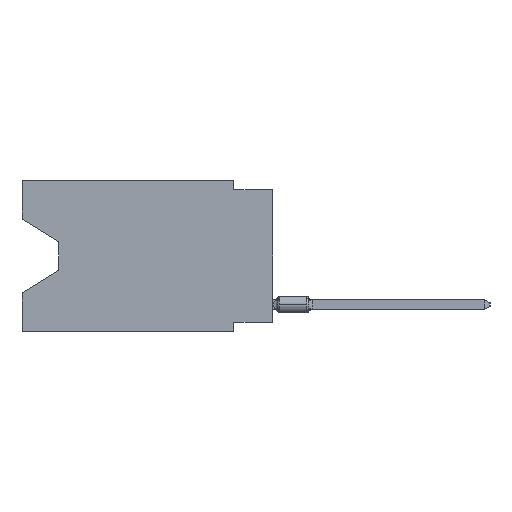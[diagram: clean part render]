
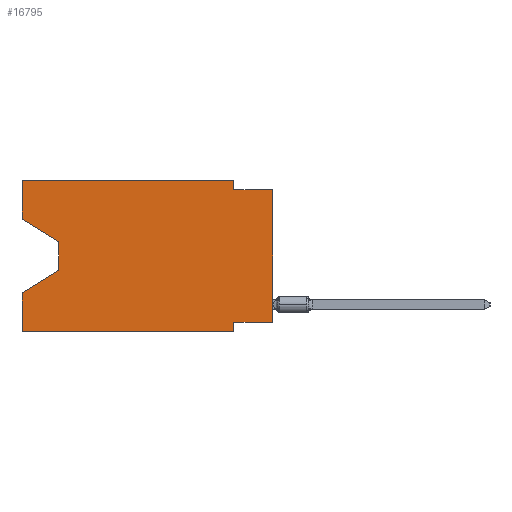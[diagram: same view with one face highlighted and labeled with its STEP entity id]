
A CAD part, left-side view. The second image highlights one B-rep face of the part: STEP entity #16795.
In plain terms, the highlighted planar face has unit normal (-1, 0, 0).
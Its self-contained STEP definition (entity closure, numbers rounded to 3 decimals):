
#233 = CARTESIAN_POINT ( 'NONE',  ( 0., 0., -0.635 ) ) ;
#667 = DIRECTION ( 'NONE',  ( 0., 0., -1. ) ) ;
#679 = EDGE_CURVE ( 'NONE', #49592, #24781, #42733, .T. ) ;
#1948 = CARTESIAN_POINT ( 'NONE',  ( 0., 16.383, -9.906 ) ) ;
#2974 = VERTEX_POINT ( 'NONE', #40757 ) ;
#4372 = CARTESIAN_POINT ( 'NONE',  ( 0., 0., -0.635 ) ) ;
#4913 = CARTESIAN_POINT ( 'NONE',  ( 0., 16.383, -9.906 ) ) ;
#5333 = CARTESIAN_POINT ( 'NONE',  ( 0., 16.383, -7.36 ) ) ;
#5532 = VECTOR ( 'NONE', #49295, 1000. ) ;
#6837 = ORIENTED_EDGE ( 'NONE', *, *, #34905, .T. ) ;
#8085 = ORIENTED_EDGE ( 'NONE', *, *, #13207, .F. ) ;
#9167 = VERTEX_POINT ( 'NONE', #4372 ) ;
#9658 = DIRECTION ( 'NONE',  ( 0., 0.855, -0.519 ) ) ;
#9728 = DIRECTION ( 'NONE',  ( 1., 0., 0. ) ) ;
#9980 = VERTEX_POINT ( 'NONE', #48731 ) ;
#10377 = CARTESIAN_POINT ( 'NONE',  ( 0., 0., -9.271 ) ) ;
#10813 = CARTESIAN_POINT ( 'NONE',  ( 0., 2.54, 0. ) ) ;
#10932 = EDGE_CURVE ( 'NONE', #11700, #13028, #24825, .T. ) ;
#11700 = VERTEX_POINT ( 'NONE', #32693 ) ;
#12869 = AXIS2_PLACEMENT_3D ( 'NONE', #33815, #9728, #41316 ) ;
#13028 = VERTEX_POINT ( 'NONE', #39754 ) ;
#13207 = EDGE_CURVE ( 'NONE', #2974, #11700, #15308, .T. ) ;
#13869 = EDGE_CURVE ( 'NONE', #2974, #36355, #14857, .T. ) ;
#14140 = ORIENTED_EDGE ( 'NONE', *, *, #16106, .T. ) ;
#14520 = DIRECTION ( 'NONE',  ( 0., 1., 0. ) ) ;
#14585 = CARTESIAN_POINT ( 'NONE',  ( 0., 2.54, -9.271 ) ) ;
#14857 = LINE ( 'NONE', #30928, #41698 ) ;
#15308 = LINE ( 'NONE', #50995, #43223 ) ;
#15534 = VECTOR ( 'NONE', #20163, 1000. ) ;
#16106 = EDGE_CURVE ( 'NONE', #34280, #16692, #37375, .T. ) ;
#16692 = VERTEX_POINT ( 'NONE', #5333 ) ;
#16795 = ADVANCED_FACE ( 'NONE', ( #18021 ), #45201, .F. ) ;
#16933 = VERTEX_POINT ( 'NONE', #4913 ) ;
#16961 = EDGE_CURVE ( 'NONE', #24781, #9980, #17344, .T. ) ;
#17344 = LINE ( 'NONE', #29515, #23800 ) ;
#17737 = LINE ( 'NONE', #1948, #5532 ) ;
#17823 = CARTESIAN_POINT ( 'NONE',  ( 0., 16.383, 0. ) ) ;
#18021 = FACE_OUTER_BOUND ( 'NONE', #45787, .T. ) ;
#18171 = ORIENTED_EDGE ( 'NONE', *, *, #49308, .F. ) ;
#18261 = VECTOR ( 'NONE', #40857, 1000. ) ;
#18980 = ORIENTED_EDGE ( 'NONE', *, *, #36967, .T. ) ;
#19524 = DIRECTION ( 'NONE',  ( 0., -0.855, -0.519 ) ) ;
#19616 = LINE ( 'NONE', #10813, #43940 ) ;
#19864 = LINE ( 'NONE', #34903, #28237 ) ;
#20163 = DIRECTION ( 'NONE',  ( 0., -1., 0. ) ) ;
#20347 = LINE ( 'NONE', #34678, #38235 ) ;
#21173 = CARTESIAN_POINT ( 'NONE',  ( 0., 13.97, -5.893 ) ) ;
#22469 = VECTOR ( 'NONE', #44544, 1000. ) ;
#23520 = DIRECTION ( 'NONE',  ( 0., 0., -1. ) ) ;
#23800 = VECTOR ( 'NONE', #40896, 1000. ) ;
#24781 = VERTEX_POINT ( 'NONE', #14585 ) ;
#24825 = LINE ( 'NONE', #17823, #18261 ) ;
#28237 = VECTOR ( 'NONE', #39286, 1000. ) ;
#28252 = ORIENTED_EDGE ( 'NONE', *, *, #10932, .F. ) ;
#28335 = ORIENTED_EDGE ( 'NONE', *, *, #45895, .F. ) ;
#28752 = CARTESIAN_POINT ( 'NONE',  ( 0., 0., 0. ) ) ;
#29515 = CARTESIAN_POINT ( 'NONE',  ( 0., 2.54, -9.906 ) ) ;
#30928 = CARTESIAN_POINT ( 'NONE',  ( 0., 16.383, -2.546 ) ) ;
#32116 = DIRECTION ( 'NONE',  ( 0., 0., 1. ) ) ;
#32264 = ORIENTED_EDGE ( 'NONE', *, *, #33635, .T. ) ;
#32693 = CARTESIAN_POINT ( 'NONE',  ( 0., 16.383, 0. ) ) ;
#33106 = ORIENTED_EDGE ( 'NONE', *, *, #16961, .F. ) ;
#33635 = EDGE_CURVE ( 'NONE', #36355, #34280, #20347, .T. ) ;
#33815 = CARTESIAN_POINT ( 'NONE',  ( 0., 16.383, 0. ) ) ;
#34280 = VERTEX_POINT ( 'NONE', #21173 ) ;
#34678 = CARTESIAN_POINT ( 'NONE',  ( 0., 13.97, -4.013 ) ) ;
#34903 = CARTESIAN_POINT ( 'NONE',  ( 0., 16.383, 0. ) ) ;
#34905 = EDGE_CURVE ( 'NONE', #16933, #9980, #17737, .T. ) ;
#35952 = LINE ( 'NONE', #233, #15534 ) ;
#36355 = VERTEX_POINT ( 'NONE', #42826 ) ;
#36967 = EDGE_CURVE ( 'NONE', #49592, #9167, #40662, .T. ) ;
#37375 = LINE ( 'NONE', #45133, #49211 ) ;
#37906 = ORIENTED_EDGE ( 'NONE', *, *, #49272, .F. ) ;
#38235 = VECTOR ( 'NONE', #667, 1000. ) ;
#38294 = ORIENTED_EDGE ( 'NONE', *, *, #679, .F. ) ;
#38487 = VECTOR ( 'NONE', #14520, 1000. ) ;
#39286 = DIRECTION ( 'NONE',  ( 0., 0., 1. ) ) ;
#39754 = CARTESIAN_POINT ( 'NONE',  ( 0., 2.54, 0. ) ) ;
#40662 = LINE ( 'NONE', #28752, #22469 ) ;
#40757 = CARTESIAN_POINT ( 'NONE',  ( 0., 16.383, -2.546 ) ) ;
#40857 = DIRECTION ( 'NONE',  ( 0., -1., 0. ) ) ;
#40896 = DIRECTION ( 'NONE',  ( 0., 0., -1. ) ) ;
#41316 = DIRECTION ( 'NONE',  ( 0., 0., -1. ) ) ;
#41698 = VECTOR ( 'NONE', #19524, 1000. ) ;
#42733 = LINE ( 'NONE', #10377, #38487 ) ;
#42826 = CARTESIAN_POINT ( 'NONE',  ( 0., 13.97, -4.013 ) ) ;
#43223 = VECTOR ( 'NONE', #32116, 1000. ) ;
#43940 = VECTOR ( 'NONE', #23520, 1000. ) ;
#44544 = DIRECTION ( 'NONE',  ( 0., 0., 1. ) ) ;
#45133 = CARTESIAN_POINT ( 'NONE',  ( 0., 13.97, -5.893 ) ) ;
#45201 = PLANE ( 'NONE',  #12869 ) ;
#45787 = EDGE_LOOP ( 'NONE', ( #48199, #32264, #14140, #18171, #6837, #33106, #38294, #18980, #28335, #37906, #28252, #8085 ) ) ;
#45895 = EDGE_CURVE ( 'NONE', #50633, #9167, #35952, .T. ) ;
#48199 = ORIENTED_EDGE ( 'NONE', *, *, #13869, .T. ) ;
#48731 = CARTESIAN_POINT ( 'NONE',  ( 0., 2.54, -9.906 ) ) ;
#49211 = VECTOR ( 'NONE', #9658, 1000. ) ;
#49272 = EDGE_CURVE ( 'NONE', #13028, #50633, #19616, .T. ) ;
#49295 = DIRECTION ( 'NONE',  ( 0., -1., 0. ) ) ;
#49308 = EDGE_CURVE ( 'NONE', #16933, #16692, #19864, .T. ) ;
#49334 = CARTESIAN_POINT ( 'NONE',  ( 0., 0., -9.271 ) ) ;
#49592 = VERTEX_POINT ( 'NONE', #49334 ) ;
#50341 = CARTESIAN_POINT ( 'NONE',  ( 0., 2.54, -0.635 ) ) ;
#50633 = VERTEX_POINT ( 'NONE', #50341 ) ;
#50995 = CARTESIAN_POINT ( 'NONE',  ( 0., 16.383, 0. ) ) ;
